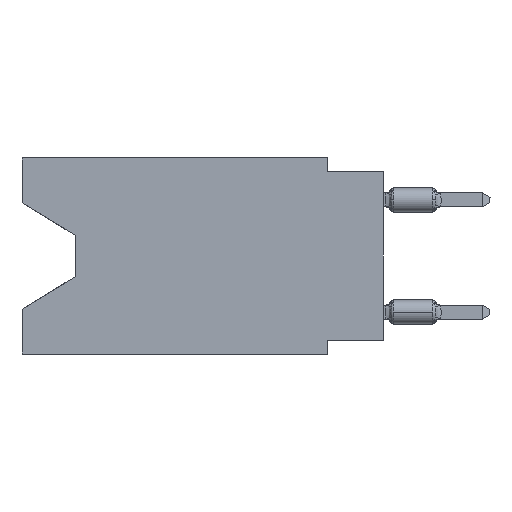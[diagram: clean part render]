
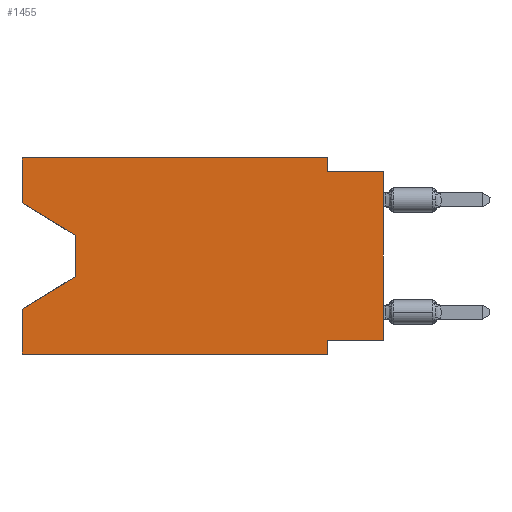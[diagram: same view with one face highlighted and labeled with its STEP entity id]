
A CAD part, left-side view. The second image highlights one B-rep face of the part: STEP entity #1455.
In plain terms, the highlighted planar face has unit normal (-1, 0, 0).
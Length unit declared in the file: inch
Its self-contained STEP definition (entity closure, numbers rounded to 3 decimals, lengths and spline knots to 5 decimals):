
#984 = VECTOR ( 'NONE', #25853, 39.37008 ) ;
#986 = DIRECTION ( 'NONE',  ( 0., 0., -1. ) ) ;
#1455 = ADVANCED_FACE ( 'NONE', ( #23119 ), #26620, .F. ) ;
#2401 = CARTESIAN_POINT ( 'NONE',  ( 0., 0.645, 0. ) ) ;
#3388 = CARTESIAN_POINT ( 'NONE',  ( 0., 0.645, -0.26975 ) ) ;
#6072 = CARTESIAN_POINT ( 'NONE',  ( 0., 0.645, -0.35 ) ) ;
#6343 = CARTESIAN_POINT ( 'NONE',  ( 0., 0.1, -0.35 ) ) ;
#7129 = VERTEX_POINT ( 'NONE', #51683 ) ;
#7225 = CARTESIAN_POINT ( 'NONE',  ( 0., 0.645, -0.08025 ) ) ;
#7867 = AXIS2_PLACEMENT_3D ( 'NONE', #2401, #43022, #13982 ) ;
#8060 = DIRECTION ( 'NONE',  ( 0., 0., 1. ) ) ;
#8916 = CARTESIAN_POINT ( 'NONE',  ( 0., 0.645, -0.08025 ) ) ;
#10195 = VECTOR ( 'NONE', #53113, 39.37008 ) ;
#10276 = VECTOR ( 'NONE', #31853, 39.37008 ) ;
#11407 = EDGE_CURVE ( 'NONE', #52337, #32964, #40889, .T. ) ;
#11419 = VERTEX_POINT ( 'NONE', #37386 ) ;
#11973 = CARTESIAN_POINT ( 'NONE',  ( 0., 0., -0.325 ) ) ;
#12288 = ORIENTED_EDGE ( 'NONE', *, *, #34114, .F. ) ;
#12488 = DIRECTION ( 'NONE',  ( 0., 0., -1. ) ) ;
#12885 = VECTOR ( 'NONE', #8060, 39.37008 ) ;
#12983 = ORIENTED_EDGE ( 'NONE', *, *, #25886, .T. ) ;
#13882 = LINE ( 'NONE', #37830, #24125 ) ;
#13982 = DIRECTION ( 'NONE',  ( 0., 0., -1. ) ) ;
#14935 = DIRECTION ( 'NONE',  ( 0., 0., 1. ) ) ;
#15565 = LINE ( 'NONE', #27407, #36374 ) ;
#15661 = ORIENTED_EDGE ( 'NONE', *, *, #24537, .F. ) ;
#15844 = LINE ( 'NONE', #36789, #36908 ) ;
#16286 = ORIENTED_EDGE ( 'NONE', *, *, #51058, .F. ) ;
#16318 = VERTEX_POINT ( 'NONE', #8916 ) ;
#18036 = VECTOR ( 'NONE', #14935, 39.37008 ) ;
#19015 = EDGE_CURVE ( 'NONE', #16318, #27893, #32481, .T. ) ;
#19349 = CARTESIAN_POINT ( 'NONE',  ( 0., 0.1, 0. ) ) ;
#21379 = ORIENTED_EDGE ( 'NONE', *, *, #29652, .T. ) ;
#21418 = CARTESIAN_POINT ( 'NONE',  ( 0., 0., -0.325 ) ) ;
#22568 = EDGE_CURVE ( 'NONE', #46586, #36361, #15565, .T. ) ;
#23119 = FACE_OUTER_BOUND ( 'NONE', #48083, .T. ) ;
#23647 = DIRECTION ( 'NONE',  ( 0., -1., 0. ) ) ;
#24125 = VECTOR ( 'NONE', #986, 39.37008 ) ;
#24537 = EDGE_CURVE ( 'NONE', #51806, #32964, #50911, .T. ) ;
#25815 = ORIENTED_EDGE ( 'NONE', *, *, #34253, .F. ) ;
#25853 = DIRECTION ( 'NONE',  ( 0., 0.855, -0.519 ) ) ;
#25886 = EDGE_CURVE ( 'NONE', #34937, #44547, #50308, .T. ) ;
#26620 = PLANE ( 'NONE',  #7867 ) ;
#27043 = DIRECTION ( 'NONE',  ( 0., -1., 0. ) ) ;
#27407 = CARTESIAN_POINT ( 'NONE',  ( 0., 0.645, 0. ) ) ;
#27585 = LINE ( 'NONE', #11973, #10195 ) ;
#27893 = VERTEX_POINT ( 'NONE', #33528 ) ;
#28606 = LINE ( 'NONE', #45291, #37089 ) ;
#29652 = EDGE_CURVE ( 'NONE', #11419, #30792, #31340, .T. ) ;
#30278 = CARTESIAN_POINT ( 'NONE',  ( 0., 0., -0.025 ) ) ;
#30301 = CARTESIAN_POINT ( 'NONE',  ( 0., 0.645, 0. ) ) ;
#30792 = VERTEX_POINT ( 'NONE', #6343 ) ;
#31015 = CARTESIAN_POINT ( 'NONE',  ( 0., 0., -0.025 ) ) ;
#31061 = CARTESIAN_POINT ( 'NONE',  ( 0., 0.645, 0. ) ) ;
#31340 = LINE ( 'NONE', #6072, #52777 ) ;
#31853 = DIRECTION ( 'NONE',  ( 0., 0., 1. ) ) ;
#32065 = ORIENTED_EDGE ( 'NONE', *, *, #48183, .F. ) ;
#32379 = CARTESIAN_POINT ( 'NONE',  ( 0., 0.645, 0. ) ) ;
#32481 = LINE ( 'NONE', #7225, #34410 ) ;
#32964 = VERTEX_POINT ( 'NONE', #30278 ) ;
#33380 = CARTESIAN_POINT ( 'NONE',  ( 0., 0.55, -0.212 ) ) ;
#33528 = CARTESIAN_POINT ( 'NONE',  ( 0., 0.55, -0.138 ) ) ;
#34114 = EDGE_CURVE ( 'NONE', #11419, #44547, #46943, .T. ) ;
#34253 = EDGE_CURVE ( 'NONE', #16318, #46586, #43960, .T. ) ;
#34410 = VECTOR ( 'NONE', #49157, 39.37008 ) ;
#34937 = VERTEX_POINT ( 'NONE', #40929 ) ;
#35333 = EDGE_CURVE ( 'NONE', #7129, #30792, #15844, .T. ) ;
#36361 = VERTEX_POINT ( 'NONE', #19349 ) ;
#36374 = VECTOR ( 'NONE', #23647, 39.37008 ) ;
#36789 = CARTESIAN_POINT ( 'NONE',  ( 0., 0.1, -0.35 ) ) ;
#36908 = VECTOR ( 'NONE', #52401, 39.37008 ) ;
#37089 = VECTOR ( 'NONE', #12488, 39.37008 ) ;
#37386 = CARTESIAN_POINT ( 'NONE',  ( 0., 0.645, -0.35 ) ) ;
#37830 = CARTESIAN_POINT ( 'NONE',  ( 0., 0.1, 0. ) ) ;
#39593 = EDGE_CURVE ( 'NONE', #27893, #34937, #28606, .T. ) ;
#40863 = ORIENTED_EDGE ( 'NONE', *, *, #11407, .T. ) ;
#40889 = LINE ( 'NONE', #49206, #12885 ) ;
#40929 = CARTESIAN_POINT ( 'NONE',  ( 0., 0.55, -0.212 ) ) ;
#43022 = DIRECTION ( 'NONE',  ( 1., 0., 0. ) ) ;
#43164 = ORIENTED_EDGE ( 'NONE', *, *, #19015, .T. ) ;
#43960 = LINE ( 'NONE', #32379, #10276 ) ;
#44240 = VECTOR ( 'NONE', #50641, 39.37008 ) ;
#44547 = VERTEX_POINT ( 'NONE', #3388 ) ;
#45016 = ORIENTED_EDGE ( 'NONE', *, *, #22568, .F. ) ;
#45291 = CARTESIAN_POINT ( 'NONE',  ( 0., 0.55, -0.138 ) ) ;
#46586 = VERTEX_POINT ( 'NONE', #30301 ) ;
#46691 = ORIENTED_EDGE ( 'NONE', *, *, #35333, .F. ) ;
#46943 = LINE ( 'NONE', #31061, #18036 ) ;
#48083 = EDGE_LOOP ( 'NONE', ( #43164, #51098, #12983, #12288, #21379, #46691, #32065, #40863, #15661, #16286, #45016, #25815 ) ) ;
#48183 = EDGE_CURVE ( 'NONE', #52337, #7129, #27585, .T. ) ;
#49157 = DIRECTION ( 'NONE',  ( 0., -0.855, -0.519 ) ) ;
#49206 = CARTESIAN_POINT ( 'NONE',  ( 0., 0., 0. ) ) ;
#50308 = LINE ( 'NONE', #33380, #984 ) ;
#50641 = DIRECTION ( 'NONE',  ( 0., -1., 0. ) ) ;
#50911 = LINE ( 'NONE', #31015, #44240 ) ;
#51054 = CARTESIAN_POINT ( 'NONE',  ( 0., 0.1, -0.025 ) ) ;
#51058 = EDGE_CURVE ( 'NONE', #36361, #51806, #13882, .T. ) ;
#51098 = ORIENTED_EDGE ( 'NONE', *, *, #39593, .T. ) ;
#51683 = CARTESIAN_POINT ( 'NONE',  ( 0., 0.1, -0.325 ) ) ;
#51806 = VERTEX_POINT ( 'NONE', #51054 ) ;
#52337 = VERTEX_POINT ( 'NONE', #21418 ) ;
#52401 = DIRECTION ( 'NONE',  ( 0., 0., -1. ) ) ;
#52777 = VECTOR ( 'NONE', #27043, 39.37008 ) ;
#53113 = DIRECTION ( 'NONE',  ( 0., 1., 0. ) ) ;
